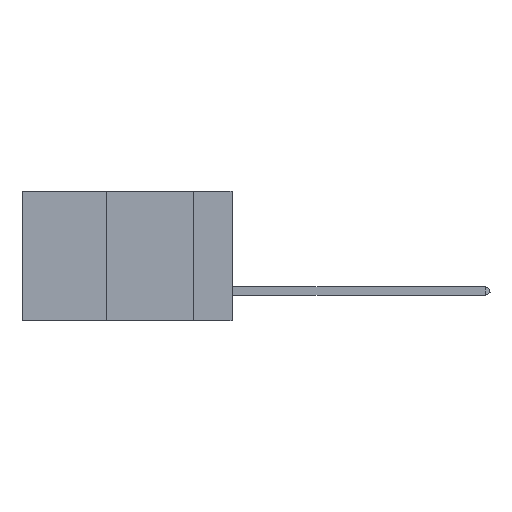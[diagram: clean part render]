
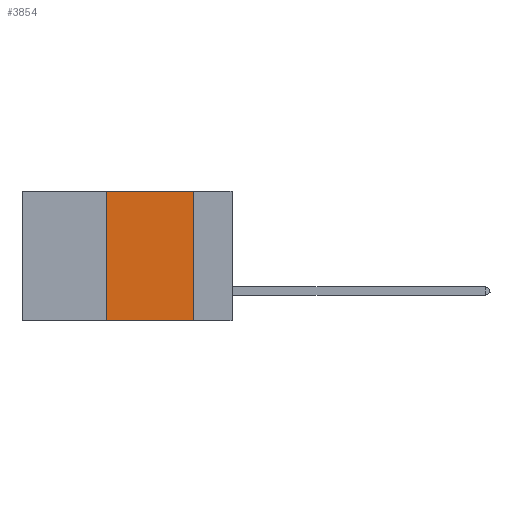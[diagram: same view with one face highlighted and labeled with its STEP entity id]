
A CAD part, left-side view. The second image highlights one B-rep face of the part: STEP entity #3854.
In plain terms, the highlighted planar face has unit normal (-1, 0, 0).
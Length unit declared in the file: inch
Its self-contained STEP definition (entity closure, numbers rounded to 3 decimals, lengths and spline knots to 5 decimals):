
#460 = CARTESIAN_POINT ( 'NONE',  ( 0., 0.6, 0. ) ) ;
#1393 = DIRECTION ( 'NONE',  ( 0., 0., -1. ) ) ;
#1655 = CARTESIAN_POINT ( 'NONE',  ( 0., 0.6, 0. ) ) ;
#2426 = EDGE_CURVE ( 'NONE', #13544, #10472, #11168, .T. ) ;
#3854 = ADVANCED_FACE ( 'NONE', ( #16007 ), #22353, .F. ) ;
#4689 = DIRECTION ( 'NONE',  ( 0., 0., 1. ) ) ;
#5240 = CARTESIAN_POINT ( 'NONE',  ( 0., 0.36, 0. ) ) ;
#5862 = ORIENTED_EDGE ( 'NONE', *, *, #2426, .F. ) ;
#6437 = CARTESIAN_POINT ( 'NONE',  ( 0., 0.36, 0. ) ) ;
#6821 = VECTOR ( 'NONE', #23085, 39.37008 ) ;
#7186 = DIRECTION ( 'NONE',  ( 0., -1., 0. ) ) ;
#7590 = EDGE_CURVE ( 'NONE', #16854, #10280, #19584, .T. ) ;
#9578 = EDGE_CURVE ( 'NONE', #13544, #10280, #12064, .T. ) ;
#9755 = CARTESIAN_POINT ( 'NONE',  ( 0., 0.11, -0.37 ) ) ;
#10280 = VERTEX_POINT ( 'NONE', #9755 ) ;
#10472 = VERTEX_POINT ( 'NONE', #6437 ) ;
#10733 = DIRECTION ( 'NONE',  ( 0., 0., -1. ) ) ;
#10869 = VECTOR ( 'NONE', #7186, 39.37008 ) ;
#11168 = LINE ( 'NONE', #5240, #14602 ) ;
#11858 = DIRECTION ( 'NONE',  ( 1., 0., 0. ) ) ;
#12064 = LINE ( 'NONE', #26804, #10869 ) ;
#12598 = LINE ( 'NONE', #460, #6821 ) ;
#12599 = CARTESIAN_POINT ( 'NONE',  ( 0., 0.36, -0.37 ) ) ;
#12818 = CARTESIAN_POINT ( 'NONE',  ( 0., 0.11, 0. ) ) ;
#13019 = ORIENTED_EDGE ( 'NONE', *, *, #7590, .F. ) ;
#13544 = VERTEX_POINT ( 'NONE', #12599 ) ;
#13858 = AXIS2_PLACEMENT_3D ( 'NONE', #1655, #11858, #1393 ) ;
#14602 = VECTOR ( 'NONE', #4689, 39.37008 ) ;
#15791 = CARTESIAN_POINT ( 'NONE',  ( 0., 0.11, 0. ) ) ;
#16007 = FACE_OUTER_BOUND ( 'NONE', #22020, .T. ) ;
#16854 = VERTEX_POINT ( 'NONE', #15791 ) ;
#17259 = ORIENTED_EDGE ( 'NONE', *, *, #9578, .T. ) ;
#18278 = VECTOR ( 'NONE', #10733, 39.37008 ) ;
#19584 = LINE ( 'NONE', #12818, #18278 ) ;
#19760 = EDGE_CURVE ( 'NONE', #10472, #16854, #12598, .T. ) ;
#20348 = ORIENTED_EDGE ( 'NONE', *, *, #19760, .F. ) ;
#22020 = EDGE_LOOP ( 'NONE', ( #13019, #20348, #5862, #17259 ) ) ;
#22353 = PLANE ( 'NONE',  #13858 ) ;
#23085 = DIRECTION ( 'NONE',  ( 0., -1., 0. ) ) ;
#26804 = CARTESIAN_POINT ( 'NONE',  ( 0., 0.6, -0.37 ) ) ;
